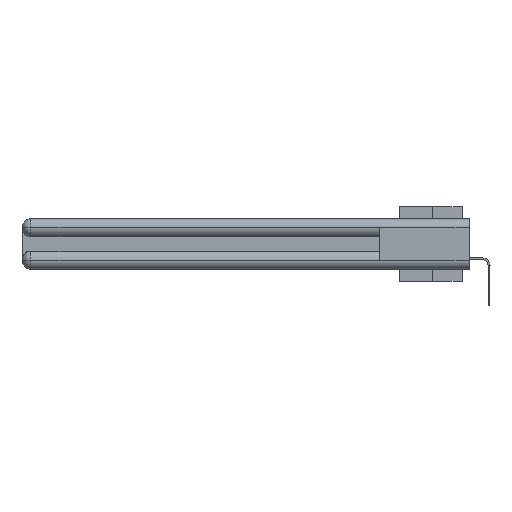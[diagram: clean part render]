
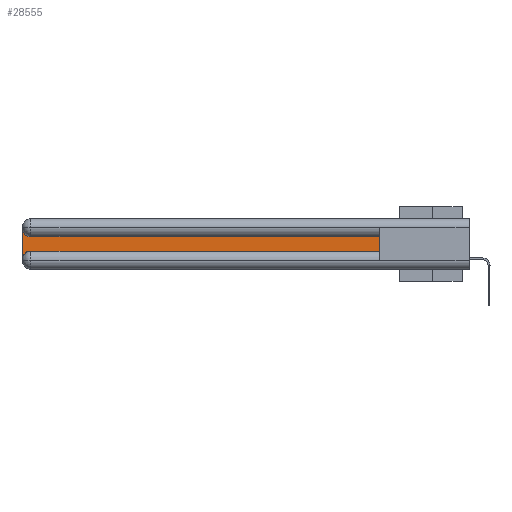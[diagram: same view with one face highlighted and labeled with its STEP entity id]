
A CAD part, left-side view. The second image highlights one B-rep face of the part: STEP entity #28555.
In plain terms, the highlighted planar face has unit normal (-1, 0, 0).
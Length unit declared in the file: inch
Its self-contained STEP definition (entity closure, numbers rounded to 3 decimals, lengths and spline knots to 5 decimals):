
#346 = EDGE_CURVE ( 'NONE', #32134, #7276, #32462, .T. ) ;
#717 = AXIS2_PLACEMENT_3D ( 'NONE', #29317, #15740, #26830 ) ;
#1410 = CARTESIAN_POINT ( 'NONE',  ( 0.075, 3., -0.2775 ) ) ;
#1627 = CARTESIAN_POINT ( 'NONE',  ( 0.075, 3., -0.1225 ) ) ;
#2532 = AXIS2_PLACEMENT_3D ( 'NONE', #1627, #4115, #22453 ) ;
#4115 = DIRECTION ( 'NONE',  ( 1., 0., 0. ) ) ;
#4465 = CARTESIAN_POINT ( 'NONE',  ( 0.075, 2.94, -0.1225 ) ) ;
#4982 = ORIENTED_EDGE ( 'NONE', *, *, #346, .T. ) ;
#5145 = CARTESIAN_POINT ( 'NONE',  ( 0.075, 0.6, -0.1225 ) ) ;
#5379 = CARTESIAN_POINT ( 'NONE',  ( 0.075, 3., -0.0625 ) ) ;
#5939 = CARTESIAN_POINT ( 'NONE',  ( 0.075, 2.94, -0.2775 ) ) ;
#6043 = DIRECTION ( 'NONE',  ( 1., 0., 0. ) ) ;
#6958 = DIRECTION ( 'NONE',  ( 0., -1., 0. ) ) ;
#7276 = VERTEX_POINT ( 'NONE', #5379 ) ;
#7358 = LINE ( 'NONE', #23061, #25995 ) ;
#7601 = ORIENTED_EDGE ( 'NONE', *, *, #11753, .T. ) ;
#8081 = LINE ( 'NONE', #5145, #11046 ) ;
#9864 = VERTEX_POINT ( 'NONE', #27037 ) ;
#10031 = VECTOR ( 'NONE', #26562, 39.37008 ) ;
#11046 = VECTOR ( 'NONE', #27238, 39.37008 ) ;
#11753 = EDGE_CURVE ( 'NONE', #9864, #32134, #8081, .T. ) ;
#14981 = DIRECTION ( 'NONE',  ( 0., 0., -1. ) ) ;
#15740 = DIRECTION ( 'NONE',  ( 1., 0., 0. ) ) ;
#17108 = LINE ( 'NONE', #25740, #17936 ) ;
#17936 = VECTOR ( 'NONE', #14981, 39.37008 ) ;
#19030 = EDGE_CURVE ( 'NONE', #19249, #26770, #28136, .T. ) ;
#19249 = VERTEX_POINT ( 'NONE', #1410 ) ;
#19280 = EDGE_CURVE ( 'NONE', #26770, #24582, #7358, .T. ) ;
#20318 = CARTESIAN_POINT ( 'NONE',  ( 0.075, 2.94, -0.2175 ) ) ;
#21823 = ORIENTED_EDGE ( 'NONE', *, *, #19280, .T. ) ;
#22453 = DIRECTION ( 'NONE',  ( 0., 0., -1. ) ) ;
#23061 = CARTESIAN_POINT ( 'NONE',  ( 0.075, 0.6, -0.2175 ) ) ;
#24144 = DIRECTION ( 'NONE',  ( 0., 0., -1. ) ) ;
#24582 = VERTEX_POINT ( 'NONE', #28228 ) ;
#24726 = FACE_OUTER_BOUND ( 'NONE', #24855, .T. ) ;
#24855 = EDGE_LOOP ( 'NONE', ( #7601, #4982, #33268, #32046, #21823, #34197 ) ) ;
#25740 = CARTESIAN_POINT ( 'NONE',  ( 0.075, 3., -0.2175 ) ) ;
#25861 = PLANE ( 'NONE',  #2532 ) ;
#25995 = VECTOR ( 'NONE', #6958, 39.37008 ) ;
#26562 = DIRECTION ( 'NONE',  ( 0., 0., 1. ) ) ;
#26770 = VERTEX_POINT ( 'NONE', #20318 ) ;
#26830 = DIRECTION ( 'NONE',  ( 0., 0., -1. ) ) ;
#26954 = EDGE_CURVE ( 'NONE', #24582, #9864, #35020, .T. ) ;
#27037 = CARTESIAN_POINT ( 'NONE',  ( 0.075, 0.6, -0.1225 ) ) ;
#27238 = DIRECTION ( 'NONE',  ( 0., 1., 0. ) ) ;
#28136 = CIRCLE ( 'NONE', #30410, 0.06 ) ;
#28228 = CARTESIAN_POINT ( 'NONE',  ( 0.075, 0.6, -0.2175 ) ) ;
#28555 = ADVANCED_FACE ( 'NONE', ( #24726 ), #25861, .F. ) ;
#29059 = CARTESIAN_POINT ( 'NONE',  ( 0.075, 0.6, -0.2175 ) ) ;
#29317 = CARTESIAN_POINT ( 'NONE',  ( 0.075, 2.94, -0.0625 ) ) ;
#30410 = AXIS2_PLACEMENT_3D ( 'NONE', #5939, #6043, #24144 ) ;
#32046 = ORIENTED_EDGE ( 'NONE', *, *, #19030, .T. ) ;
#32134 = VERTEX_POINT ( 'NONE', #4465 ) ;
#32462 = CIRCLE ( 'NONE', #717, 0.06 ) ;
#33268 = ORIENTED_EDGE ( 'NONE', *, *, #34024, .T. ) ;
#34024 = EDGE_CURVE ( 'NONE', #7276, #19249, #17108, .T. ) ;
#34197 = ORIENTED_EDGE ( 'NONE', *, *, #26954, .T. ) ;
#35020 = LINE ( 'NONE', #29059, #10031 ) ;
